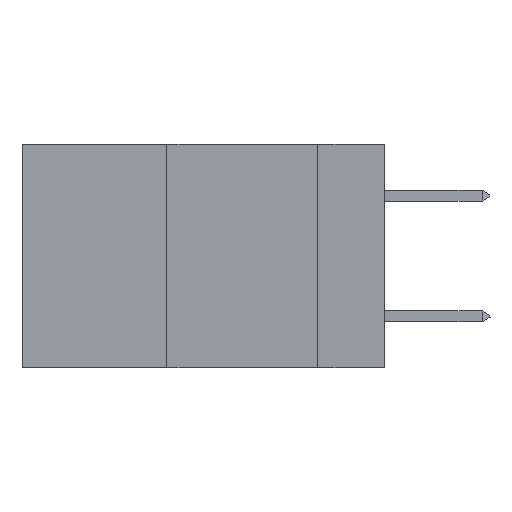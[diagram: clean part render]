
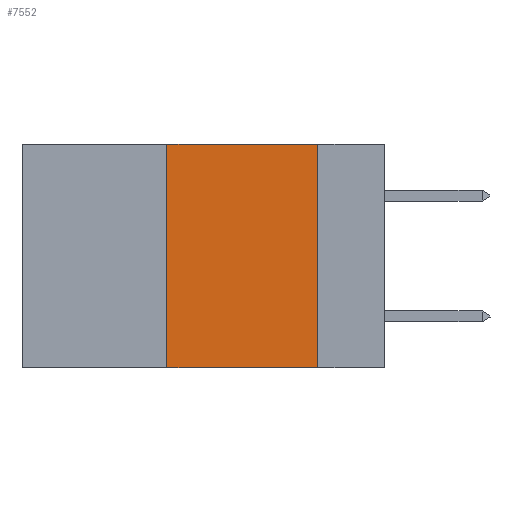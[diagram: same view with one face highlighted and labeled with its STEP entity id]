
A CAD part, left-side view. The second image highlights one B-rep face of the part: STEP entity #7552.
In plain terms, the highlighted planar face has unit normal (-1, 0, 0).
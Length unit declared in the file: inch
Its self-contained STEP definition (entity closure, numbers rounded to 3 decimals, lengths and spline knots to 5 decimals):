
#317 = CARTESIAN_POINT ( 'NONE',  ( 0., 0.11, -0.37 ) ) ;
#583 = CARTESIAN_POINT ( 'NONE',  ( 0., 0.11, 0. ) ) ;
#809 = EDGE_CURVE ( 'NONE', #6089, #11759, #9378, .T. ) ;
#992 = ORIENTED_EDGE ( 'NONE', *, *, #809, .T. ) ;
#1144 = EDGE_LOOP ( 'NONE', ( #5146, #11733, #5059, #992 ) ) ;
#1192 = VECTOR ( 'NONE', #1715, 39.37008 ) ;
#1715 = DIRECTION ( 'NONE',  ( 0., -1., 0. ) ) ;
#2557 = VERTEX_POINT ( 'NONE', #5810 ) ;
#2665 = VECTOR ( 'NONE', #5943, 39.37008 ) ;
#2861 = EDGE_CURVE ( 'NONE', #6089, #9762, #8635, .T. ) ;
#5059 = ORIENTED_EDGE ( 'NONE', *, *, #2861, .F. ) ;
#5075 = FACE_OUTER_BOUND ( 'NONE', #1144, .T. ) ;
#5146 = ORIENTED_EDGE ( 'NONE', *, *, #5234, .F. ) ;
#5234 = EDGE_CURVE ( 'NONE', #2557, #11759, #6862, .T. ) ;
#5333 = LINE ( 'NONE', #14228, #13142 ) ;
#5810 = CARTESIAN_POINT ( 'NONE',  ( 0., 0.11, 0. ) ) ;
#5943 = DIRECTION ( 'NONE',  ( 0., 0., -1. ) ) ;
#6089 = VERTEX_POINT ( 'NONE', #11053 ) ;
#6149 = DIRECTION ( 'NONE',  ( 0., 0., 1. ) ) ;
#6862 = LINE ( 'NONE', #583, #2665 ) ;
#7204 = CARTESIAN_POINT ( 'NONE',  ( 0., 0.36, 0. ) ) ;
#7552 = ADVANCED_FACE ( 'NONE', ( #5075 ), #14094, .F. ) ;
#7635 = AXIS2_PLACEMENT_3D ( 'NONE', #10857, #9124, #11887 ) ;
#8635 = LINE ( 'NONE', #7204, #9810 ) ;
#9124 = DIRECTION ( 'NONE',  ( 1., 0., 0. ) ) ;
#9378 = LINE ( 'NONE', #10570, #1192 ) ;
#9387 = CARTESIAN_POINT ( 'NONE',  ( 0., 0.36, 0. ) ) ;
#9762 = VERTEX_POINT ( 'NONE', #9387 ) ;
#9810 = VECTOR ( 'NONE', #6149, 39.37008 ) ;
#10570 = CARTESIAN_POINT ( 'NONE',  ( 0., 0.6, -0.37 ) ) ;
#10857 = CARTESIAN_POINT ( 'NONE',  ( 0., 0.6, 0. ) ) ;
#11053 = CARTESIAN_POINT ( 'NONE',  ( 0., 0.36, -0.37 ) ) ;
#11733 = ORIENTED_EDGE ( 'NONE', *, *, #12591, .F. ) ;
#11759 = VERTEX_POINT ( 'NONE', #317 ) ;
#11887 = DIRECTION ( 'NONE',  ( 0., 0., -1. ) ) ;
#12591 = EDGE_CURVE ( 'NONE', #9762, #2557, #5333, .T. ) ;
#13142 = VECTOR ( 'NONE', #13614, 39.37008 ) ;
#13614 = DIRECTION ( 'NONE',  ( 0., -1., 0. ) ) ;
#14094 = PLANE ( 'NONE',  #7635 ) ;
#14228 = CARTESIAN_POINT ( 'NONE',  ( 0., 0.6, 0. ) ) ;
